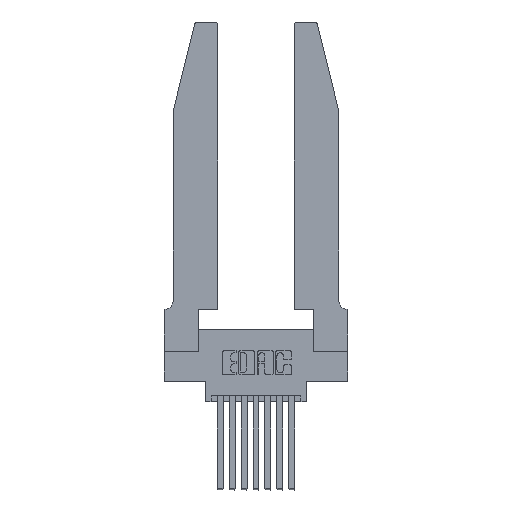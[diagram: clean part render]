
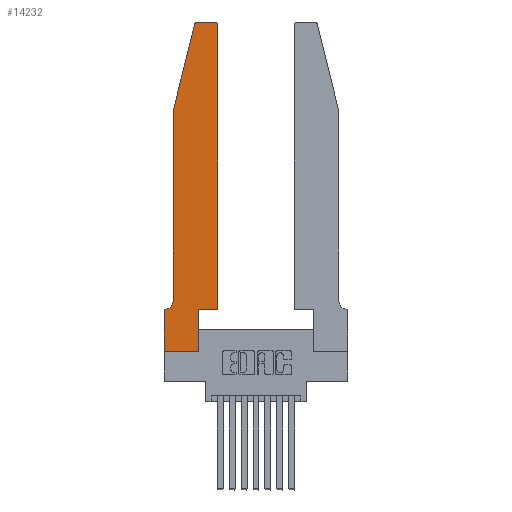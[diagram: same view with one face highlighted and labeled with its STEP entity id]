
A CAD part, top view. The second image highlights one B-rep face of the part: STEP entity #14232.
In plain terms, the highlighted planar face has unit normal (0, 0, 1).
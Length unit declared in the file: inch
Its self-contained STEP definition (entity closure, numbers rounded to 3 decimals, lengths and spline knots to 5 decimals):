
#312 = DIRECTION ( 'NONE',  ( -1., 0., 0. ) ) ;
#448 = CARTESIAN_POINT ( 'NONE',  ( 0.284, 2.75, 0.37 ) ) ;
#550 = CARTESIAN_POINT ( 'NONE',  ( 0.4505, 0.35, 0.37 ) ) ;
#795 = CARTESIAN_POINT ( 'NONE',  ( 0., 0., 0.37 ) ) ;
#836 = ORIENTED_EDGE ( 'NONE', *, *, #10871, .T. ) ;
#880 = VERTEX_POINT ( 'NONE', #6992 ) ;
#951 = ORIENTED_EDGE ( 'NONE', *, *, #2869, .T. ) ;
#983 = DIRECTION ( 'NONE',  ( 1., 0., 0. ) ) ;
#1008 = VERTEX_POINT ( 'NONE', #550 ) ;
#1079 = CARTESIAN_POINT ( 'NONE',  ( 0.4505, 0.35, 0.37 ) ) ;
#1098 = FACE_OUTER_BOUND ( 'NONE', #14145, .T. ) ;
#1152 = VERTEX_POINT ( 'NONE', #6249 ) ;
#1272 = DIRECTION ( 'NONE',  ( 0., -1., 0. ) ) ;
#2006 = CARTESIAN_POINT ( 'NONE',  ( 0.0755, 2., 0.37 ) ) ;
#2095 = CARTESIAN_POINT ( 'NONE',  ( 0.0755, 0.35, 0.37 ) ) ;
#2115 = EDGE_CURVE ( 'NONE', #2547, #2812, #10686, .T. ) ;
#2348 = ORIENTED_EDGE ( 'NONE', *, *, #9404, .T. ) ;
#2547 = VERTEX_POINT ( 'NONE', #4487 ) ;
#2595 = DIRECTION ( 'NONE',  ( 1., 0., 0. ) ) ;
#2613 = DIRECTION ( 'NONE',  ( 0., 0., 1. ) ) ;
#2646 = LINE ( 'NONE', #795, #14331 ) ;
#2805 = LINE ( 'NONE', #9767, #14138 ) ;
#2812 = VERTEX_POINT ( 'NONE', #10915 ) ;
#2869 = EDGE_CURVE ( 'NONE', #10949, #14164, #4106, .T. ) ;
#3411 = AXIS2_PLACEMENT_3D ( 'NONE', #6825, #14623, #7963 ) ;
#3749 = VERTEX_POINT ( 'NONE', #10753 ) ;
#4106 = CIRCLE ( 'NONE', #10322, 0.03 ) ;
#4362 = CARTESIAN_POINT ( 'NONE',  ( 0.284, 2.72, 0.37 ) ) ;
#4476 = LINE ( 'NONE', #10534, #13071 ) ;
#4487 = CARTESIAN_POINT ( 'NONE',  ( 0.0755, 0.42, 0.37 ) ) ;
#4491 = EDGE_CURVE ( 'NONE', #1008, #10756, #6619, .T. ) ;
#5117 = EDGE_CURVE ( 'NONE', #880, #1008, #5189, .T. ) ;
#5189 = LINE ( 'NONE', #1079, #10792 ) ;
#5477 = ORIENTED_EDGE ( 'NONE', *, *, #11997, .T. ) ;
#6051 = CARTESIAN_POINT ( 'NONE',  ( 0.2865, 0.35, 0.37 ) ) ;
#6085 = CARTESIAN_POINT ( 'NONE',  ( 0., 0.35, 0.37 ) ) ;
#6249 = CARTESIAN_POINT ( 'NONE',  ( 0.4205, 2.75, 0.37 ) ) ;
#6577 = EDGE_CURVE ( 'NONE', #2812, #11713, #11090, .T. ) ;
#6619 = LINE ( 'NONE', #9850, #9252 ) ;
#6677 = DIRECTION ( 'NONE',  ( 0., 0., -1. ) ) ;
#6694 = DIRECTION ( 'NONE',  ( -1., 0., 0. ) ) ;
#6726 = CARTESIAN_POINT ( 'NONE',  ( 0.0055, 0.42, 0.37 ) ) ;
#6825 = CARTESIAN_POINT ( 'NONE',  ( 0.4205, 2.72, 0.37 ) ) ;
#6992 = CARTESIAN_POINT ( 'NONE',  ( 0.2865, 0.35, 0.37 ) ) ;
#6997 = CARTESIAN_POINT ( 'NONE',  ( 0.4505, 2.72, 0.37 ) ) ;
#7159 = DIRECTION ( 'NONE',  ( 1., 0., 0. ) ) ;
#7219 = DIRECTION ( 'NONE',  ( 1., 0., 0. ) ) ;
#7368 = ORIENTED_EDGE ( 'NONE', *, *, #2115, .T. ) ;
#7520 = VECTOR ( 'NONE', #8905, 39.37008 ) ;
#7703 = ORIENTED_EDGE ( 'NONE', *, *, #8600, .T. ) ;
#7799 = VECTOR ( 'NONE', #13460, 39.37008 ) ;
#7890 = CIRCLE ( 'NONE', #3411, 0.03 ) ;
#7963 = DIRECTION ( 'NONE',  ( 1., 0., 0. ) ) ;
#8307 = PLANE ( 'NONE',  #9069 ) ;
#8600 = EDGE_CURVE ( 'NONE', #3749, #11708, #2646, .T. ) ;
#8844 = CARTESIAN_POINT ( 'NONE',  ( 0., 0.35, 0.37 ) ) ;
#8905 = DIRECTION ( 'NONE',  ( -0.239, -0.971, 0. ) ) ;
#8945 = EDGE_CURVE ( 'NONE', #14164, #11375, #13451, .T. ) ;
#9069 = AXIS2_PLACEMENT_3D ( 'NONE', #6085, #13904, #7219 ) ;
#9252 = VECTOR ( 'NONE', #10036, 39.37008 ) ;
#9398 = AXIS2_PLACEMENT_3D ( 'NONE', #6726, #6677, #6694 ) ;
#9404 = EDGE_CURVE ( 'NONE', #1152, #10949, #2805, .T. ) ;
#9463 = ORIENTED_EDGE ( 'NONE', *, *, #10233, .T. ) ;
#9526 = ORIENTED_EDGE ( 'NONE', *, *, #8945, .T. ) ;
#9572 = ORIENTED_EDGE ( 'NONE', *, *, #6577, .T. ) ;
#9580 = ORIENTED_EDGE ( 'NONE', *, *, #5117, .T. ) ;
#9767 = CARTESIAN_POINT ( 'NONE',  ( 0.2605, 2.75, 0.37 ) ) ;
#9850 = CARTESIAN_POINT ( 'NONE',  ( 0.4505, 0.35, 0.37 ) ) ;
#10036 = DIRECTION ( 'NONE',  ( 0., 1., 0. ) ) ;
#10233 = EDGE_CURVE ( 'NONE', #11375, #2547, #4476, .T. ) ;
#10322 = AXIS2_PLACEMENT_3D ( 'NONE', #4362, #2613, #2595 ) ;
#10534 = CARTESIAN_POINT ( 'NONE',  ( 0.0755, 2., 0.37 ) ) ;
#10570 = ORIENTED_EDGE ( 'NONE', *, *, #4491, .T. ) ;
#10686 = CIRCLE ( 'NONE', #9398, 0.07 ) ;
#10753 = CARTESIAN_POINT ( 'NONE',  ( 0., 0., 0.37 ) ) ;
#10756 = VERTEX_POINT ( 'NONE', #6997 ) ;
#10767 = LINE ( 'NONE', #14920, #13381 ) ;
#10792 = VECTOR ( 'NONE', #983, 39.37008 ) ;
#10861 = ORIENTED_EDGE ( 'NONE', *, *, #14459, .T. ) ;
#10871 = EDGE_CURVE ( 'NONE', #11708, #880, #11331, .T. ) ;
#10915 = CARTESIAN_POINT ( 'NONE',  ( 0.0055, 0.35, 0.37 ) ) ;
#10949 = VERTEX_POINT ( 'NONE', #448 ) ;
#11090 = LINE ( 'NONE', #2095, #7799 ) ;
#11331 = LINE ( 'NONE', #6051, #14291 ) ;
#11375 = VERTEX_POINT ( 'NONE', #13778 ) ;
#11708 = VERTEX_POINT ( 'NONE', #14398 ) ;
#11713 = VERTEX_POINT ( 'NONE', #8844 ) ;
#11997 = EDGE_CURVE ( 'NONE', #11713, #3749, #10767, .T. ) ;
#13071 = VECTOR ( 'NONE', #14935, 39.37008 ) ;
#13381 = VECTOR ( 'NONE', #1272, 39.37008 ) ;
#13451 = LINE ( 'NONE', #2006, #7520 ) ;
#13460 = DIRECTION ( 'NONE',  ( -1., 0., 0. ) ) ;
#13758 = CARTESIAN_POINT ( 'NONE',  ( 0.25487, 2.72718, 0.37 ) ) ;
#13778 = CARTESIAN_POINT ( 'NONE',  ( 0.0755, 2., 0.37 ) ) ;
#13824 = DIRECTION ( 'NONE',  ( 0., 1., 0. ) ) ;
#13904 = DIRECTION ( 'NONE',  ( 0., 0., 1. ) ) ;
#14138 = VECTOR ( 'NONE', #312, 39.37008 ) ;
#14145 = EDGE_LOOP ( 'NONE', ( #2348, #951, #9526, #9463, #7368, #9572, #5477, #7703, #836, #9580, #10570, #10861 ) ) ;
#14164 = VERTEX_POINT ( 'NONE', #13758 ) ;
#14232 = ADVANCED_FACE ( 'NONE', ( #1098 ), #8307, .T. ) ;
#14291 = VECTOR ( 'NONE', #13824, 39.37008 ) ;
#14331 = VECTOR ( 'NONE', #7159, 39.37008 ) ;
#14398 = CARTESIAN_POINT ( 'NONE',  ( 0.2865, 0., 0.37 ) ) ;
#14459 = EDGE_CURVE ( 'NONE', #10756, #1152, #7890, .T. ) ;
#14623 = DIRECTION ( 'NONE',  ( 0., 0., 1. ) ) ;
#14920 = CARTESIAN_POINT ( 'NONE',  ( 0., 0., 0.37 ) ) ;
#14935 = DIRECTION ( 'NONE',  ( 0., -1., 0. ) ) ;
